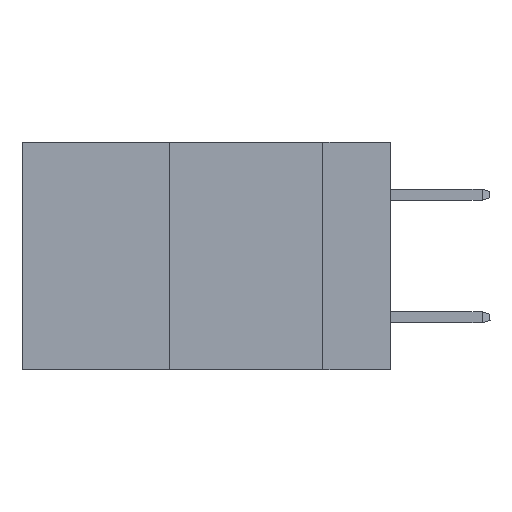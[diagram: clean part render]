
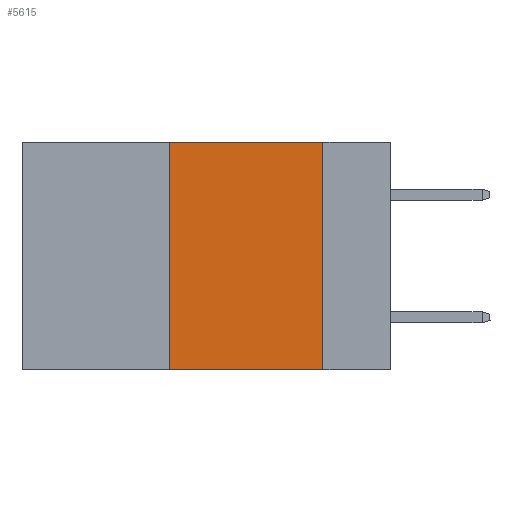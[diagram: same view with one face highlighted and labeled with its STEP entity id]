
A CAD part, left-side view. The second image highlights one B-rep face of the part: STEP entity #5615.
In plain terms, the highlighted planar face has unit normal (-1, 0, 0).
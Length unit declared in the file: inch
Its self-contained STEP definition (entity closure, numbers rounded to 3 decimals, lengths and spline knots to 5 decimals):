
#223 = ORIENTED_EDGE ( 'NONE', *, *, #11656, .F. ) ;
#280 = ORIENTED_EDGE ( 'NONE', *, *, #1844, .F. ) ;
#294 = ORIENTED_EDGE ( 'NONE', *, *, #5188, .F. ) ;
#333 = ORIENTED_EDGE ( 'NONE', *, *, #11393, .T. ) ;
#1481 = CARTESIAN_POINT ( 'NONE',  ( 0., 0.36, 0. ) ) ;
#1796 = CARTESIAN_POINT ( 'NONE',  ( 0., 0.11, 0. ) ) ;
#1844 = EDGE_CURVE ( 'NONE', #4082, #4005, #6684, .T. ) ;
#2667 = CARTESIAN_POINT ( 'NONE',  ( 0., 0.36, 0. ) ) ;
#2841 = CARTESIAN_POINT ( 'NONE',  ( 0., 0.6, 0. ) ) ;
#2920 = CARTESIAN_POINT ( 'NONE',  ( 0., 0.6, 0. ) ) ;
#3046 = VECTOR ( 'NONE', #10653, 39.37008 ) ;
#4005 = VERTEX_POINT ( 'NONE', #6060 ) ;
#4082 = VERTEX_POINT ( 'NONE', #2667 ) ;
#4780 = PLANE ( 'NONE',  #5041 ) ;
#5041 = AXIS2_PLACEMENT_3D ( 'NONE', #2841, #10911, #5719 ) ;
#5188 = EDGE_CURVE ( 'NONE', #6357, #4082, #6185, .T. ) ;
#5256 = EDGE_LOOP ( 'NONE', ( #223, #280, #294, #333 ) ) ;
#5615 = ADVANCED_FACE ( 'NONE', ( #6573 ), #4780, .F. ) ;
#5719 = DIRECTION ( 'NONE',  ( 0., 0., -1. ) ) ;
#6060 = CARTESIAN_POINT ( 'NONE',  ( 0., 0.11, 0. ) ) ;
#6185 = LINE ( 'NONE', #1481, #3046 ) ;
#6357 = VERTEX_POINT ( 'NONE', #11278 ) ;
#6450 = DIRECTION ( 'NONE',  ( 0., 0., -1. ) ) ;
#6485 = LINE ( 'NONE', #8873, #6759 ) ;
#6573 = FACE_OUTER_BOUND ( 'NONE', #5256, .T. ) ;
#6684 = LINE ( 'NONE', #2920, #6959 ) ;
#6759 = VECTOR ( 'NONE', #8014, 39.37008 ) ;
#6959 = VECTOR ( 'NONE', #10327, 39.37008 ) ;
#7158 = LINE ( 'NONE', #1796, #9433 ) ;
#7987 = VERTEX_POINT ( 'NONE', #11574 ) ;
#8014 = DIRECTION ( 'NONE',  ( 0., -1., 0. ) ) ;
#8873 = CARTESIAN_POINT ( 'NONE',  ( 0., 0.6, -0.37 ) ) ;
#9433 = VECTOR ( 'NONE', #6450, 39.37008 ) ;
#10327 = DIRECTION ( 'NONE',  ( 0., -1., 0. ) ) ;
#10653 = DIRECTION ( 'NONE',  ( 0., 0., 1. ) ) ;
#10911 = DIRECTION ( 'NONE',  ( 1., 0., 0. ) ) ;
#11278 = CARTESIAN_POINT ( 'NONE',  ( 0., 0.36, -0.37 ) ) ;
#11393 = EDGE_CURVE ( 'NONE', #6357, #7987, #6485, .T. ) ;
#11574 = CARTESIAN_POINT ( 'NONE',  ( 0., 0.11, -0.37 ) ) ;
#11656 = EDGE_CURVE ( 'NONE', #4005, #7987, #7158, .T. ) ;
